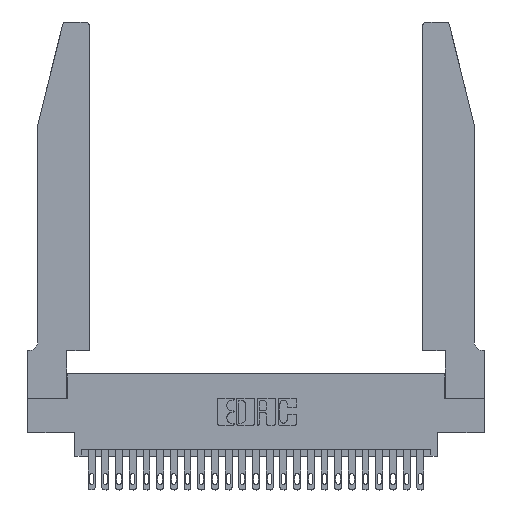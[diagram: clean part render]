
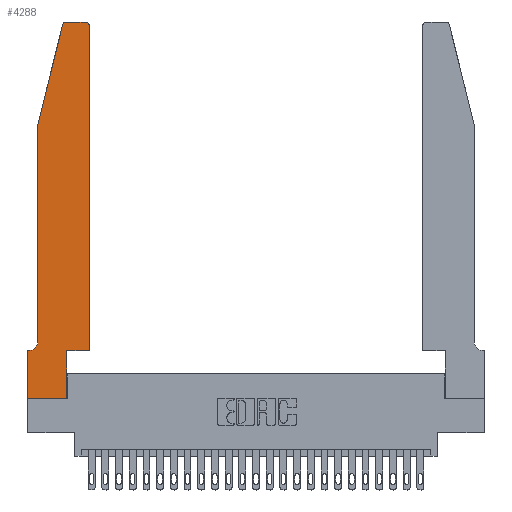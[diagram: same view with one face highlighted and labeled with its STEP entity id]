
A CAD part, top view. The second image highlights one B-rep face of the part: STEP entity #4288.
In plain terms, the highlighted planar face has unit normal (0, 0, 1).
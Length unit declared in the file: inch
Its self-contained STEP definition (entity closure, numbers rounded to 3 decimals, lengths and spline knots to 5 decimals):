
#874 = DIRECTION ( 'NONE',  ( -1., 0., 0. ) ) ;
#1157 = CARTESIAN_POINT ( 'NONE',  ( 0.4505, 2.72, 0.37 ) ) ;
#1206 = ORIENTED_EDGE ( 'NONE', *, *, #11486, .T. ) ;
#1214 = CARTESIAN_POINT ( 'NONE',  ( 0.2865, 0.35, 0.37 ) ) ;
#1381 = CARTESIAN_POINT ( 'NONE',  ( 0., 0., 0.37 ) ) ;
#1384 = CARTESIAN_POINT ( 'NONE',  ( 0.4505, 0.35, 0.37 ) ) ;
#1483 = CARTESIAN_POINT ( 'NONE',  ( 0.4205, 2.75, 0.37 ) ) ;
#1618 = CIRCLE ( 'NONE', #7366, 0.03 ) ;
#2012 = LINE ( 'NONE', #14322, #9458 ) ;
#2150 = EDGE_CURVE ( 'NONE', #10218, #23660, #12463, .T. ) ;
#2424 = LINE ( 'NONE', #3473, #11476 ) ;
#2687 = LINE ( 'NONE', #11101, #6233 ) ;
#2900 = CARTESIAN_POINT ( 'NONE',  ( 0.4505, 0.35, 0.37 ) ) ;
#3058 = PLANE ( 'NONE',  #7609 ) ;
#3236 = DIRECTION ( 'NONE',  ( 1., 0., 0. ) ) ;
#3473 = CARTESIAN_POINT ( 'NONE',  ( 0., 0., 0.37 ) ) ;
#3726 = ORIENTED_EDGE ( 'NONE', *, *, #20995, .T. ) ;
#4288 = ADVANCED_FACE ( 'NONE', ( #19729 ), #3058, .T. ) ;
#4425 = VECTOR ( 'NONE', #14245, 39.37008 ) ;
#4432 = DIRECTION ( 'NONE',  ( 0., 0., -1. ) ) ;
#4598 = CARTESIAN_POINT ( 'NONE',  ( 0., 0.35, 0.37 ) ) ;
#4844 = VECTOR ( 'NONE', #19354, 39.37008 ) ;
#5104 = VERTEX_POINT ( 'NONE', #4598 ) ;
#5680 = CARTESIAN_POINT ( 'NONE',  ( 0.284, 2.75, 0.37 ) ) ;
#5727 = VECTOR ( 'NONE', #26370, 39.37008 ) ;
#5973 = VECTOR ( 'NONE', #18046, 39.37008 ) ;
#6233 = VECTOR ( 'NONE', #15140, 39.37008 ) ;
#6417 = ORIENTED_EDGE ( 'NONE', *, *, #17295, .T. ) ;
#6459 = ORIENTED_EDGE ( 'NONE', *, *, #7966, .T. ) ;
#7366 = AXIS2_PLACEMENT_3D ( 'NONE', #15606, #15780, #3236 ) ;
#7474 = CARTESIAN_POINT ( 'NONE',  ( 0.4205, 2.72, 0.37 ) ) ;
#7609 = AXIS2_PLACEMENT_3D ( 'NONE', #21591, #9299, #11470 ) ;
#7966 = EDGE_CURVE ( 'NONE', #23711, #18749, #16693, .T. ) ;
#8232 = CARTESIAN_POINT ( 'NONE',  ( 0., 0., 0.37 ) ) ;
#8258 = CIRCLE ( 'NONE', #18408, 0.03 ) ;
#8445 = ORIENTED_EDGE ( 'NONE', *, *, #21847, .T. ) ;
#9061 = VERTEX_POINT ( 'NONE', #5680 ) ;
#9299 = DIRECTION ( 'NONE',  ( 0., 0., 1. ) ) ;
#9458 = VECTOR ( 'NONE', #24676, 39.37008 ) ;
#9692 = ORIENTED_EDGE ( 'NONE', *, *, #2150, .T. ) ;
#9916 = ORIENTED_EDGE ( 'NONE', *, *, #25396, .T. ) ;
#10218 = VERTEX_POINT ( 'NONE', #26184 ) ;
#10266 = LINE ( 'NONE', #16061, #4425 ) ;
#10939 = ORIENTED_EDGE ( 'NONE', *, *, #15883, .T. ) ;
#11101 = CARTESIAN_POINT ( 'NONE',  ( 0.0755, 2., 0.37 ) ) ;
#11220 = AXIS2_PLACEMENT_3D ( 'NONE', #16782, #4432, #18812 ) ;
#11470 = DIRECTION ( 'NONE',  ( 1., 0., 0. ) ) ;
#11476 = VECTOR ( 'NONE', #26197, 39.37008 ) ;
#11486 = EDGE_CURVE ( 'NONE', #23660, #5104, #18768, .T. ) ;
#12210 = CARTESIAN_POINT ( 'NONE',  ( 0.0755, 2., 0.37 ) ) ;
#12463 = CIRCLE ( 'NONE', #11220, 0.07 ) ;
#12482 = VERTEX_POINT ( 'NONE', #20522 ) ;
#12849 = EDGE_CURVE ( 'NONE', #9061, #22776, #1618, .T. ) ;
#13213 = LINE ( 'NONE', #25021, #16758 ) ;
#13317 = EDGE_CURVE ( 'NONE', #19979, #10218, #13213, .T. ) ;
#13813 = VERTEX_POINT ( 'NONE', #1483 ) ;
#14145 = CARTESIAN_POINT ( 'NONE',  ( 0.4505, 0.35, 0.37 ) ) ;
#14245 = DIRECTION ( 'NONE',  ( 0., 1., 0. ) ) ;
#14322 = CARTESIAN_POINT ( 'NONE',  ( 0.2605, 2.75, 0.37 ) ) ;
#14791 = CARTESIAN_POINT ( 'NONE',  ( 0.25487, 2.72718, 0.37 ) ) ;
#14909 = VERTEX_POINT ( 'NONE', #8232 ) ;
#15140 = DIRECTION ( 'NONE',  ( -0.239, -0.971, 0. ) ) ;
#15606 = CARTESIAN_POINT ( 'NONE',  ( 0.284, 2.72, 0.37 ) ) ;
#15780 = DIRECTION ( 'NONE',  ( 0., 0., 1. ) ) ;
#15883 = EDGE_CURVE ( 'NONE', #23115, #13813, #8258, .T. ) ;
#16061 = CARTESIAN_POINT ( 'NONE',  ( 0.2865, 0.35, 0.37 ) ) ;
#16473 = EDGE_CURVE ( 'NONE', #5104, #14909, #18848, .T. ) ;
#16693 = LINE ( 'NONE', #1384, #5727 ) ;
#16758 = VECTOR ( 'NONE', #18874, 39.37008 ) ;
#16782 = CARTESIAN_POINT ( 'NONE',  ( 0.0055, 0.42, 0.37 ) ) ;
#17054 = ORIENTED_EDGE ( 'NONE', *, *, #13317, .T. ) ;
#17295 = EDGE_CURVE ( 'NONE', #22776, #19979, #2687, .T. ) ;
#17410 = LINE ( 'NONE', #2900, #4844 ) ;
#17618 = CARTESIAN_POINT ( 'NONE',  ( 0.0055, 0.35, 0.37 ) ) ;
#17794 = VECTOR ( 'NONE', #874, 39.37008 ) ;
#18046 = DIRECTION ( 'NONE',  ( 0., -1., 0. ) ) ;
#18408 = AXIS2_PLACEMENT_3D ( 'NONE', #7474, #26116, #21741 ) ;
#18512 = CARTESIAN_POINT ( 'NONE',  ( 0.0755, 0.35, 0.37 ) ) ;
#18749 = VERTEX_POINT ( 'NONE', #14145 ) ;
#18768 = LINE ( 'NONE', #18512, #17794 ) ;
#18812 = DIRECTION ( 'NONE',  ( -1., 0., 0. ) ) ;
#18848 = LINE ( 'NONE', #1381, #5973 ) ;
#18874 = DIRECTION ( 'NONE',  ( 0., -1., 0. ) ) ;
#19243 = EDGE_LOOP ( 'NONE', ( #8445, #25062, #6417, #17054, #9692, #1206, #24897, #9916, #26102, #6459, #3726, #10939 ) ) ;
#19354 = DIRECTION ( 'NONE',  ( 0., 1., 0. ) ) ;
#19729 = FACE_OUTER_BOUND ( 'NONE', #19243, .T. ) ;
#19979 = VERTEX_POINT ( 'NONE', #12210 ) ;
#20522 = CARTESIAN_POINT ( 'NONE',  ( 0.2865, 0., 0.37 ) ) ;
#20995 = EDGE_CURVE ( 'NONE', #18749, #23115, #17410, .T. ) ;
#21591 = CARTESIAN_POINT ( 'NONE',  ( 0., 0.35, 0.37 ) ) ;
#21741 = DIRECTION ( 'NONE',  ( 1., 0., 0. ) ) ;
#21847 = EDGE_CURVE ( 'NONE', #13813, #9061, #2012, .T. ) ;
#22506 = EDGE_CURVE ( 'NONE', #12482, #23711, #10266, .T. ) ;
#22776 = VERTEX_POINT ( 'NONE', #14791 ) ;
#23115 = VERTEX_POINT ( 'NONE', #1157 ) ;
#23660 = VERTEX_POINT ( 'NONE', #17618 ) ;
#23711 = VERTEX_POINT ( 'NONE', #1214 ) ;
#24676 = DIRECTION ( 'NONE',  ( -1., 0., 0. ) ) ;
#24897 = ORIENTED_EDGE ( 'NONE', *, *, #16473, .T. ) ;
#25021 = CARTESIAN_POINT ( 'NONE',  ( 0.0755, 2., 0.37 ) ) ;
#25062 = ORIENTED_EDGE ( 'NONE', *, *, #12849, .T. ) ;
#25396 = EDGE_CURVE ( 'NONE', #14909, #12482, #2424, .T. ) ;
#26102 = ORIENTED_EDGE ( 'NONE', *, *, #22506, .T. ) ;
#26116 = DIRECTION ( 'NONE',  ( 0., 0., 1. ) ) ;
#26184 = CARTESIAN_POINT ( 'NONE',  ( 0.0755, 0.42, 0.37 ) ) ;
#26197 = DIRECTION ( 'NONE',  ( 1., 0., 0. ) ) ;
#26370 = DIRECTION ( 'NONE',  ( 1., 0., 0. ) ) ;
